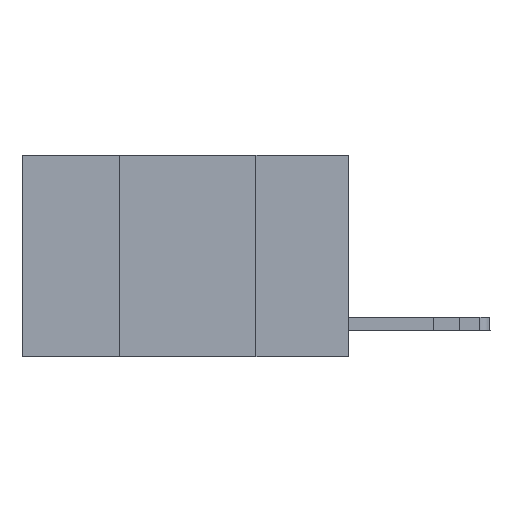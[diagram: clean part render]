
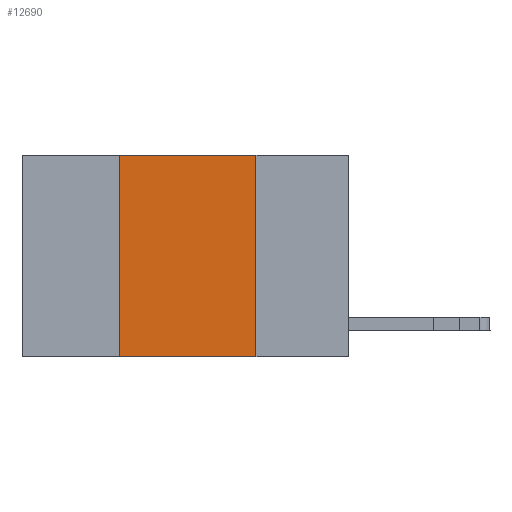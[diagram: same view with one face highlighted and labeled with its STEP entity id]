
A CAD part, left-side view. The second image highlights one B-rep face of the part: STEP entity #12690.
In plain terms, the highlighted planar face has unit normal (-1, 0, 0).
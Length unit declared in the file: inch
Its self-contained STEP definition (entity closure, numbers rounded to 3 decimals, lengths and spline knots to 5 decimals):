
#488 = CARTESIAN_POINT ( 'NONE',  ( 0., 0.17, 0. ) ) ;
#1428 = CARTESIAN_POINT ( 'NONE',  ( 0., 0.17, -0.37 ) ) ;
#1499 = LINE ( 'NONE', #3525, #13977 ) ;
#1859 = EDGE_LOOP ( 'NONE', ( #6706, #13285, #13674, #4157 ) ) ;
#1998 = EDGE_CURVE ( 'NONE', #14317, #7689, #9824, .T. ) ;
#2429 = VERTEX_POINT ( 'NONE', #9544 ) ;
#2504 = DIRECTION ( 'NONE',  ( 0., 0., -1. ) ) ;
#3086 = FACE_OUTER_BOUND ( 'NONE', #1859, .T. ) ;
#3525 = CARTESIAN_POINT ( 'NONE',  ( 0., 0.6, -0.37 ) ) ;
#4157 = ORIENTED_EDGE ( 'NONE', *, *, #7153, .T. ) ;
#4358 = VECTOR ( 'NONE', #12421, 39.37008 ) ;
#4975 = CARTESIAN_POINT ( 'NONE',  ( 0., 0.6, 0. ) ) ;
#5964 = LINE ( 'NONE', #6456, #12182 ) ;
#6456 = CARTESIAN_POINT ( 'NONE',  ( 0., 0.42, 0. ) ) ;
#6706 = ORIENTED_EDGE ( 'NONE', *, *, #9662, .F. ) ;
#7153 = EDGE_CURVE ( 'NONE', #2429, #8155, #1499, .T. ) ;
#7689 = VERTEX_POINT ( 'NONE', #488 ) ;
#8155 = VERTEX_POINT ( 'NONE', #1428 ) ;
#8345 = CARTESIAN_POINT ( 'NONE',  ( 0., 0.17, 0. ) ) ;
#8596 = CARTESIAN_POINT ( 'NONE',  ( 0., 0.42, 0. ) ) ;
#8825 = EDGE_CURVE ( 'NONE', #2429, #14317, #5964, .T. ) ;
#8964 = DIRECTION ( 'NONE',  ( 0., 0., 1. ) ) ;
#9544 = CARTESIAN_POINT ( 'NONE',  ( 0., 0.42, -0.37 ) ) ;
#9649 = VECTOR ( 'NONE', #12016, 39.37008 ) ;
#9662 = EDGE_CURVE ( 'NONE', #7689, #8155, #10029, .T. ) ;
#9824 = LINE ( 'NONE', #4975, #4358 ) ;
#9993 = DIRECTION ( 'NONE',  ( 1., 0., 0. ) ) ;
#10029 = LINE ( 'NONE', #8345, #9649 ) ;
#11182 = PLANE ( 'NONE',  #15735 ) ;
#12016 = DIRECTION ( 'NONE',  ( 0., 0., -1. ) ) ;
#12182 = VECTOR ( 'NONE', #8964, 39.37008 ) ;
#12421 = DIRECTION ( 'NONE',  ( 0., -1., 0. ) ) ;
#12690 = ADVANCED_FACE ( 'NONE', ( #3086 ), #11182, .F. ) ;
#13285 = ORIENTED_EDGE ( 'NONE', *, *, #1998, .F. ) ;
#13481 = DIRECTION ( 'NONE',  ( 0., -1., 0. ) ) ;
#13658 = CARTESIAN_POINT ( 'NONE',  ( 0., 0.6, 0. ) ) ;
#13674 = ORIENTED_EDGE ( 'NONE', *, *, #8825, .F. ) ;
#13977 = VECTOR ( 'NONE', #13481, 39.37008 ) ;
#14317 = VERTEX_POINT ( 'NONE', #8596 ) ;
#15735 = AXIS2_PLACEMENT_3D ( 'NONE', #13658, #9993, #2504 ) ;
